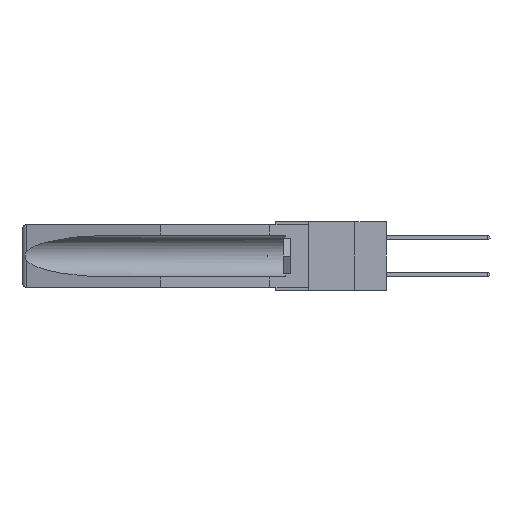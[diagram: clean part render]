
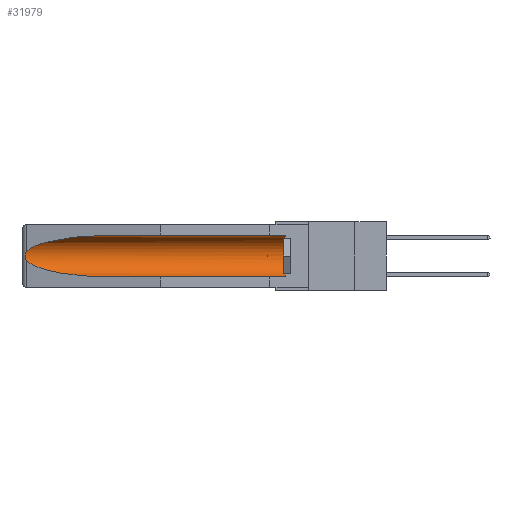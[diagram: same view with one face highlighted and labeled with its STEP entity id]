
A CAD part, left-side view. The second image highlights one B-rep face of the part: STEP entity #31979.
In plain terms, the highlighted cylindrical face has radius 2.857 mm (diameter 5.715 mm), a partial arc.
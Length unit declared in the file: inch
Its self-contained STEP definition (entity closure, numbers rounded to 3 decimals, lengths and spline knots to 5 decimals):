
#66 = CARTESIAN_POINT ( 'NONE',  ( 0.155, -0.30754, -0.284 ) ) ;
#101 = DIRECTION ( 'NONE',  ( 0., 0., 1. ) ) ;
#214 = CARTESIAN_POINT ( 'NONE',  ( 0.26537, 1.52718, -0.19328 ) ) ;
#1402 = EDGE_CURVE ( 'NONE', #17223, #13978, #10040, .T. ) ;
#1748 = CARTESIAN_POINT ( 'NONE',  ( 0.155, 1.07973, -0.284 ) ) ;
#2971 = CARTESIAN_POINT ( 'NONE',  ( 0.26597, 1.5296, -0.19026 ) ) ;
#3173 = ORIENTED_EDGE ( 'NONE', *, *, #23509, .T. ) ;
#4027 = CARTESIAN_POINT ( 'NONE',  ( 0.155, -0.30754, -0.1715 ) ) ;
#4449 = VECTOR ( 'NONE', #12146, 39.37008 ) ;
#4890 = CARTESIAN_POINT ( 'NONE',  ( 0.155, 0.126, -0.059 ) ) ;
#5598 = CARTESIAN_POINT ( 'NONE',  ( 0.26597, 1.52961, -0.15275 ) ) ;
#6502 = CARTESIAN_POINT ( 'NONE',  ( 0.155, 1.07973, -0.059 ) ) ;
#6848 = CYLINDRICAL_SURFACE ( 'NONE', #21867, 0.1125 ) ;
#7743 = EDGE_CURVE ( 'NONE', #33542, #23757, #14925, .T. ) ;
#8097 = LINE ( 'NONE', #66, #18304 ) ;
#8353 = DIRECTION ( 'NONE',  ( 0., -1., 0. ) ) ;
#8455 = CARTESIAN_POINT ( 'NONE',  ( 0.2675, 1.53308, -0.16763 ) ) ;
#10040 = CIRCLE ( 'NONE', #11987, 0.1125 ) ;
#11074 = CARTESIAN_POINT ( 'NONE',  ( 0.26655, 1.53094, -0.18657 ) ) ;
#11901 = ORIENTED_EDGE ( 'NONE', *, *, #18324, .T. ) ;
#11987 = AXIS2_PLACEMENT_3D ( 'NONE', #35154, #8353, #101 ) ;
#12146 = DIRECTION ( 'NONE',  ( 0., 1., 0. ) ) ;
#13124 = ORIENTED_EDGE ( 'NONE', *, *, #22399, .F. ) ;
#13243 = CARTESIAN_POINT ( 'NONE',  ( 0.155, 1.07973, -0.284 ) ) ;
#13285 = VERTEX_POINT ( 'NONE', #15291 ) ;
#13978 = VERTEX_POINT ( 'NONE', #4890 ) ;
#14241 = LINE ( 'NONE', #18229, #4449 ) ;
#14925 =( BOUNDED_CURVE ( )  B_SPLINE_CURVE ( 3, ( #21448, #32462, #32348, #13243 ),
 .UNSPECIFIED., .F., .F. ) 
 B_SPLINE_CURVE_WITH_KNOTS ( ( 4, 4 ),
 ( 0.1948, 1.5708 ),
 .UNSPECIFIED. ) 
 CURVE ( )  GEOMETRIC_REPRESENTATION_ITEM ( )  RATIONAL_B_SPLINE_CURVE ( ( 1., 0.848, 0.848, 1. ) ) 
 REPRESENTATION_ITEM ( '' )  );
#14989 = DIRECTION ( 'NONE',  ( 0., 1., 0. ) ) ;
#15291 = CARTESIAN_POINT ( 'NONE',  ( 0.155, 1.07973, -0.059 ) ) ;
#16546 = CARTESIAN_POINT ( 'NONE',  ( 0.26654, 1.53092, -0.15636 ) ) ;
#16625 = DIRECTION ( 'NONE',  ( 0., 1., 0. ) ) ;
#17003 = CARTESIAN_POINT ( 'NONE',  ( 0.21114, 1.30732, -0.059 ) ) ;
#17223 = VERTEX_POINT ( 'NONE', #33650 ) ;
#17342 = CARTESIAN_POINT ( 'NONE',  ( 0.26537, 1.52718, -0.14972 ) ) ;
#18229 = CARTESIAN_POINT ( 'NONE',  ( 0.155, -0.30754, -0.059 ) ) ;
#18304 = VECTOR ( 'NONE', #16625, 39.37008 ) ;
#18324 = EDGE_CURVE ( 'NONE', #13285, #20056, #18632, .T. ) ;
#18632 =( BOUNDED_CURVE ( )  B_SPLINE_CURVE ( 3, ( #6502, #17003, #28210, #17342 ),
 .UNSPECIFIED., .F., .F. ) 
 B_SPLINE_CURVE_WITH_KNOTS ( ( 4, 4 ),
 ( 4.71239, 6.08839 ),
 .UNSPECIFIED. ) 
 CURVE ( )  GEOMETRIC_REPRESENTATION_ITEM ( )  RATIONAL_B_SPLINE_CURVE ( ( 1., 0.848, 0.848, 1. ) ) 
 REPRESENTATION_ITEM ( '' )  );
#20056 = VERTEX_POINT ( 'NONE', #20327 ) ;
#20291 = ORIENTED_EDGE ( 'NONE', *, *, #1402, .T. ) ;
#20327 = CARTESIAN_POINT ( 'NONE',  ( 0.26537, 1.52718, -0.14972 ) ) ;
#20639 = EDGE_LOOP ( 'NONE', ( #11901, #3173, #29199, #13124, #20291, #23291 ) ) ;
#21448 = CARTESIAN_POINT ( 'NONE',  ( 0.26537, 1.52718, -0.19328 ) ) ;
#21867 = AXIS2_PLACEMENT_3D ( 'NONE', #4027, #14989, #26243 ) ;
#21880 = CARTESIAN_POINT ( 'NONE',  ( 0.26537, 1.52718, -0.14972 ) ) ;
#22399 = EDGE_CURVE ( 'NONE', #17223, #23757, #8097, .T. ) ;
#23291 = ORIENTED_EDGE ( 'NONE', *, *, #25961, .T. ) ;
#23307 = CARTESIAN_POINT ( 'NONE',  ( 0.26537, 1.52718, -0.19328 ) ) ;
#23509 = EDGE_CURVE ( 'NONE', #20056, #33542, #25986, .T. ) ;
#23757 = VERTEX_POINT ( 'NONE', #1748 ) ;
#24596 = CARTESIAN_POINT ( 'NONE',  ( 0.2673, 1.5327, -0.16383 ) ) ;
#25961 = EDGE_CURVE ( 'NONE', #13978, #13285, #14241, .T. ) ;
#25986 = B_SPLINE_CURVE_WITH_KNOTS ( 'NONE', 3,
 ( #21880, #5598, #16546, #24596, #8455, #27314, #27540, #11074, #2971, #214 ),
 .UNSPECIFIED., .F., .F.,
 ( 4, 2, 2, 2, 4 ),
 ( 0., 0.00029, 0.00058, 0.00087, 0.00117 ),
 .UNSPECIFIED. ) ;
#26243 = DIRECTION ( 'NONE',  ( 0., 0., 1. ) ) ;
#27314 = CARTESIAN_POINT ( 'NONE',  ( 0.2675, 1.53308, -0.17534 ) ) ;
#27540 = CARTESIAN_POINT ( 'NONE',  ( 0.2673, 1.53269, -0.17917 ) ) ;
#28210 = CARTESIAN_POINT ( 'NONE',  ( 0.25451, 1.48313, -0.09465 ) ) ;
#28494 = FACE_OUTER_BOUND ( 'NONE', #20639, .T. ) ;
#29199 = ORIENTED_EDGE ( 'NONE', *, *, #7743, .T. ) ;
#31979 = ADVANCED_FACE ( 'NONE', ( #28494 ), #6848, .F. ) ;
#32348 = CARTESIAN_POINT ( 'NONE',  ( 0.21114, 1.30732, -0.284 ) ) ;
#32462 = CARTESIAN_POINT ( 'NONE',  ( 0.25451, 1.48313, -0.24835 ) ) ;
#33542 = VERTEX_POINT ( 'NONE', #23307 ) ;
#33650 = CARTESIAN_POINT ( 'NONE',  ( 0.155, 0.126, -0.284 ) ) ;
#35154 = CARTESIAN_POINT ( 'NONE',  ( 0.155, 0.126, -0.1715 ) ) ;
